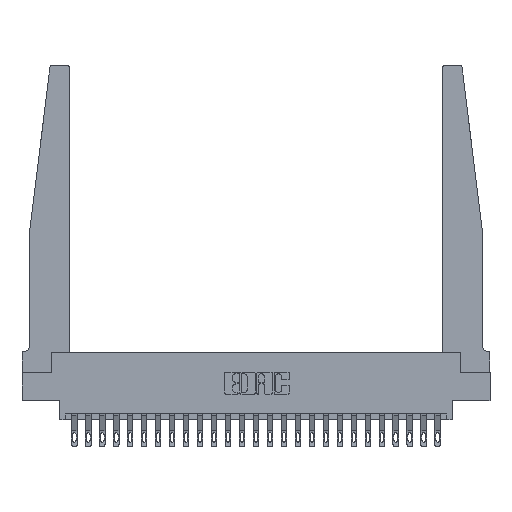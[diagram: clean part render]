
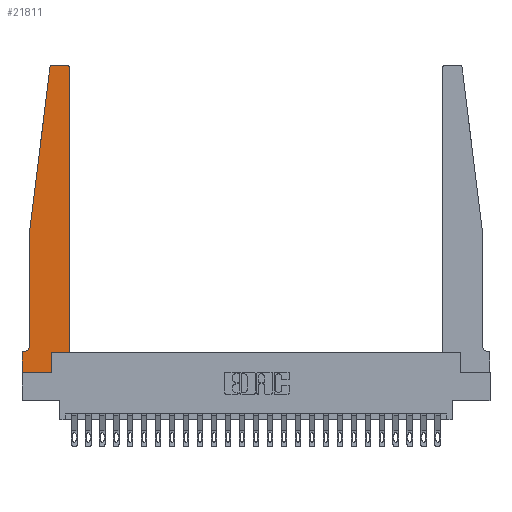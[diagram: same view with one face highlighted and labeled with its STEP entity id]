
A CAD part, top view. The second image highlights one B-rep face of the part: STEP entity #21811.
In plain terms, the highlighted planar face has unit normal (0, 0, 1).
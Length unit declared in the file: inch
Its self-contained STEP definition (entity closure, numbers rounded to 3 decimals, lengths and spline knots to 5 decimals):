
#376 = LINE ( 'NONE', #16018, #10660 ) ;
#486 = CARTESIAN_POINT ( 'NONE',  ( 0.27653, 2.75, 0.37 ) ) ;
#831 = VERTEX_POINT ( 'NONE', #22660 ) ;
#843 = VECTOR ( 'NONE', #20654, 39.37008 ) ;
#1078 = DIRECTION ( 'NONE',  ( 1., 0., 0. ) ) ;
#1205 = VERTEX_POINT ( 'NONE', #21970 ) ;
#1450 = LINE ( 'NONE', #16130, #21307 ) ;
#1545 = CARTESIAN_POINT ( 'NONE',  ( 0., 0.1875, 0.37 ) ) ;
#1906 = CARTESIAN_POINT ( 'NONE',  ( 0.425, 2.72, 0.37 ) ) ;
#2036 = AXIS2_PLACEMENT_3D ( 'NONE', #21264, #9802, #23186 ) ;
#2510 = DIRECTION ( 'NONE',  ( 0., -1., 0. ) ) ;
#2538 = ORIENTED_EDGE ( 'NONE', *, *, #4158, .T. ) ;
#2558 = DIRECTION ( 'NONE',  ( -0.122, -0.992, 0. ) ) ;
#2919 = CARTESIAN_POINT ( 'NONE',  ( 0.2605, 0., 0.37 ) ) ;
#3159 = AXIS2_PLACEMENT_3D ( 'NONE', #15517, #9807, #23194 ) ;
#4089 = LINE ( 'NONE', #15981, #18831 ) ;
#4158 = EDGE_CURVE ( 'NONE', #23903, #16091, #4831, .T. ) ;
#4747 = AXIS2_PLACEMENT_3D ( 'NONE', #8125, #21516, #10055 ) ;
#4831 = LINE ( 'NONE', #24698, #15091 ) ;
#5025 = EDGE_CURVE ( 'NONE', #6195, #24102, #1450, .T. ) ;
#5611 = DIRECTION ( 'NONE',  ( 1., 0., 0. ) ) ;
#5937 = PLANE ( 'NONE',  #3159 ) ;
#6195 = VERTEX_POINT ( 'NONE', #13906 ) ;
#6613 = LINE ( 'NONE', #14994, #843 ) ;
#7061 = ORIENTED_EDGE ( 'NONE', *, *, #17736, .T. ) ;
#7069 = CARTESIAN_POINT ( 'NONE',  ( 0.065, 0.1875, 0.37 ) ) ;
#7206 = DIRECTION ( 'NONE',  ( -1., 0., 0. ) ) ;
#7552 = ORIENTED_EDGE ( 'NONE', *, *, #17191, .T. ) ;
#7712 = VERTEX_POINT ( 'NONE', #15742 ) ;
#8125 = CARTESIAN_POINT ( 'NONE',  ( 0.27653, 2.72, 0.37 ) ) ;
#8324 = VERTEX_POINT ( 'NONE', #15477 ) ;
#8416 = VECTOR ( 'NONE', #7206, 39.37008 ) ;
#8543 = ORIENTED_EDGE ( 'NONE', *, *, #19906, .T. ) ;
#8606 = VECTOR ( 'NONE', #1078, 39.37008 ) ;
#8661 = EDGE_LOOP ( 'NONE', ( #10752, #8543, #20913, #18976, #13152, #24021, #7061, #2538, #22950, #7552, #20115, #9658 ) ) ;
#8998 = DIRECTION ( 'NONE',  ( -1., 0., 0. ) ) ;
#9003 = CIRCLE ( 'NONE', #19777, 0.05 ) ;
#9007 = EDGE_CURVE ( 'NONE', #7712, #6195, #376, .T. ) ;
#9095 = VECTOR ( 'NONE', #12816, 39.37008 ) ;
#9134 = DIRECTION ( 'NONE',  ( 0., 0., -1. ) ) ;
#9525 = LINE ( 'NONE', #7069, #19115 ) ;
#9658 = ORIENTED_EDGE ( 'NONE', *, *, #12563, .T. ) ;
#9802 = DIRECTION ( 'NONE',  ( 0., 0., 1. ) ) ;
#9807 = DIRECTION ( 'NONE',  ( 0., 0., 1. ) ) ;
#10055 = DIRECTION ( 'NONE',  ( 1., 0., 0. ) ) ;
#10660 = VECTOR ( 'NONE', #2558, 39.37008 ) ;
#10752 = ORIENTED_EDGE ( 'NONE', *, *, #14992, .T. ) ;
#10975 = CARTESIAN_POINT ( 'NONE',  ( 0.25, 2.75, 0.37 ) ) ;
#11127 = FACE_OUTER_BOUND ( 'NONE', #8661, .T. ) ;
#11353 = VERTEX_POINT ( 'NONE', #23481 ) ;
#11630 = CARTESIAN_POINT ( 'NONE',  ( 0.065, 0.2375, 0.37 ) ) ;
#11702 = VERTEX_POINT ( 'NONE', #1545 ) ;
#12271 = EDGE_CURVE ( 'NONE', #1205, #18096, #19302, .T. ) ;
#12563 = EDGE_CURVE ( 'NONE', #18096, #11353, #22871, .T. ) ;
#12816 = DIRECTION ( 'NONE',  ( 0., 1., 0. ) ) ;
#13152 = ORIENTED_EDGE ( 'NONE', *, *, #14983, .T. ) ;
#13837 = EDGE_CURVE ( 'NONE', #16091, #831, #6613, .T. ) ;
#13906 = CARTESIAN_POINT ( 'NONE',  ( 0.065, 1.25, 0.37 ) ) ;
#14983 = EDGE_CURVE ( 'NONE', #24102, #8324, #9003, .T. ) ;
#14992 = EDGE_CURVE ( 'NONE', #11353, #16983, #23684, .T. ) ;
#14994 = CARTESIAN_POINT ( 'NONE',  ( 0.2605, 0.18, 0.37 ) ) ;
#15091 = VECTOR ( 'NONE', #5611, 39.37008 ) ;
#15152 = CIRCLE ( 'NONE', #4747, 0.03 ) ;
#15477 = CARTESIAN_POINT ( 'NONE',  ( 0.015, 0.1875, 0.37 ) ) ;
#15517 = CARTESIAN_POINT ( 'NONE',  ( 0., 0.1875, 0.37 ) ) ;
#15742 = CARTESIAN_POINT ( 'NONE',  ( 0.24675, 2.72367, 0.37 ) ) ;
#15981 = CARTESIAN_POINT ( 'NONE',  ( 0., 0., 0.37 ) ) ;
#16018 = CARTESIAN_POINT ( 'NONE',  ( 0.065, 1.25, 0.37 ) ) ;
#16091 = VERTEX_POINT ( 'NONE', #2919 ) ;
#16130 = CARTESIAN_POINT ( 'NONE',  ( 0.065, 1.25, 0.37 ) ) ;
#16983 = VERTEX_POINT ( 'NONE', #486 ) ;
#17191 = EDGE_CURVE ( 'NONE', #831, #1205, #18809, .T. ) ;
#17736 = EDGE_CURVE ( 'NONE', #11702, #23903, #4089, .T. ) ;
#17979 = EDGE_CURVE ( 'NONE', #8324, #11702, #9525, .T. ) ;
#18096 = VERTEX_POINT ( 'NONE', #1906 ) ;
#18809 = LINE ( 'NONE', #24101, #8606 ) ;
#18831 = VECTOR ( 'NONE', #2510, 39.37008 ) ;
#18976 = ORIENTED_EDGE ( 'NONE', *, *, #5025, .T. ) ;
#19115 = VECTOR ( 'NONE', #8998, 39.37008 ) ;
#19302 = LINE ( 'NONE', #24280, #9095 ) ;
#19777 = AXIS2_PLACEMENT_3D ( 'NONE', #20604, #9134, #22542 ) ;
#19906 = EDGE_CURVE ( 'NONE', #16983, #7712, #15152, .T. ) ;
#20115 = ORIENTED_EDGE ( 'NONE', *, *, #12271, .T. ) ;
#20604 = CARTESIAN_POINT ( 'NONE',  ( 0.015, 0.2375, 0.37 ) ) ;
#20654 = DIRECTION ( 'NONE',  ( 0., 1., 0. ) ) ;
#20913 = ORIENTED_EDGE ( 'NONE', *, *, #9007, .T. ) ;
#21264 = CARTESIAN_POINT ( 'NONE',  ( 0.395, 2.72, 0.37 ) ) ;
#21307 = VECTOR ( 'NONE', #21898, 39.37008 ) ;
#21516 = DIRECTION ( 'NONE',  ( 0., 0., 1. ) ) ;
#21811 = ADVANCED_FACE ( 'NONE', ( #11127 ), #5937, .T. ) ;
#21898 = DIRECTION ( 'NONE',  ( 0., -1., 0. ) ) ;
#21970 = CARTESIAN_POINT ( 'NONE',  ( 0.425, 0.18, 0.37 ) ) ;
#22361 = CARTESIAN_POINT ( 'NONE',  ( 0., 0., 0.37 ) ) ;
#22542 = DIRECTION ( 'NONE',  ( -1., 0., 0. ) ) ;
#22660 = CARTESIAN_POINT ( 'NONE',  ( 0.2605, 0.18, 0.37 ) ) ;
#22871 = CIRCLE ( 'NONE', #2036, 0.03 ) ;
#22950 = ORIENTED_EDGE ( 'NONE', *, *, #13837, .T. ) ;
#23186 = DIRECTION ( 'NONE',  ( 1., 0., 0. ) ) ;
#23194 = DIRECTION ( 'NONE',  ( 1., 0., 0. ) ) ;
#23481 = CARTESIAN_POINT ( 'NONE',  ( 0.395, 2.75, 0.37 ) ) ;
#23684 = LINE ( 'NONE', #10975, #8416 ) ;
#23903 = VERTEX_POINT ( 'NONE', #22361 ) ;
#24021 = ORIENTED_EDGE ( 'NONE', *, *, #17979, .T. ) ;
#24101 = CARTESIAN_POINT ( 'NONE',  ( 0.425, 0.18, 0.37 ) ) ;
#24102 = VERTEX_POINT ( 'NONE', #11630 ) ;
#24280 = CARTESIAN_POINT ( 'NONE',  ( 0.425, 0.18, 0.37 ) ) ;
#24698 = CARTESIAN_POINT ( 'NONE',  ( 0., 0., 0.37 ) ) ;
